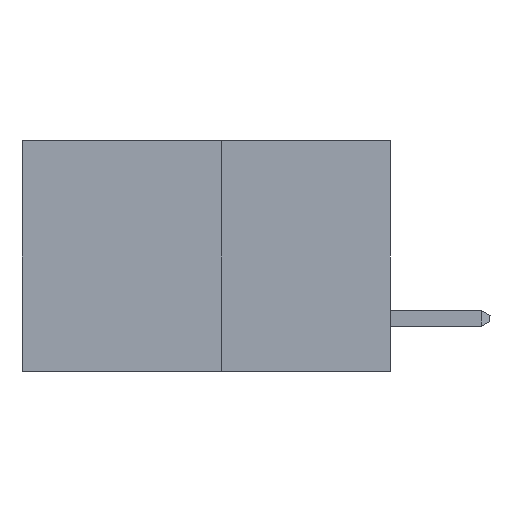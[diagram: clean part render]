
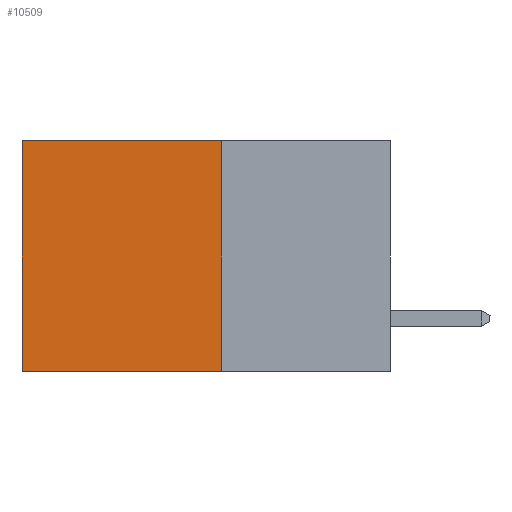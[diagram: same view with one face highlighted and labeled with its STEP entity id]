
A CAD part, left-side view. The second image highlights one B-rep face of the part: STEP entity #10509.
In plain terms, the highlighted planar face has unit normal (-1, 0, 0).
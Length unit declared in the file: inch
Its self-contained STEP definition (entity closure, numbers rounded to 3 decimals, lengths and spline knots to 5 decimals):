
#114 = CARTESIAN_POINT ( 'NONE',  ( 0.277, 0.27, -0.37 ) ) ;
#220 = EDGE_LOOP ( 'NONE', ( #13788, #3759, #4108, #1432 ) ) ;
#617 = PLANE ( 'NONE',  #11642 ) ;
#951 = CARTESIAN_POINT ( 'NONE',  ( 0.277, 0.27, -0.37 ) ) ;
#1059 = DIRECTION ( 'NONE',  ( 0., 0., -1. ) ) ;
#1062 = DIRECTION ( 'NONE',  ( 0., 1., 0. ) ) ;
#1432 = ORIENTED_EDGE ( 'NONE', *, *, #11243, .T. ) ;
#1532 = VECTOR ( 'NONE', #1059, 39.37008 ) ;
#2311 = VECTOR ( 'NONE', #1062, 39.37008 ) ;
#2806 = DIRECTION ( 'NONE',  ( 0., 1., 0. ) ) ;
#2920 = DIRECTION ( 'NONE',  ( 0., 0., -1. ) ) ;
#3384 = VERTEX_POINT ( 'NONE', #4161 ) ;
#3733 = EDGE_CURVE ( 'NONE', #11399, #3384, #7106, .T. ) ;
#3759 = ORIENTED_EDGE ( 'NONE', *, *, #3733, .F. ) ;
#4075 = VECTOR ( 'NONE', #2806, 39.37008 ) ;
#4108 = ORIENTED_EDGE ( 'NONE', *, *, #5228, .F. ) ;
#4161 = CARTESIAN_POINT ( 'NONE',  ( 0.277, 0.59, -0.37 ) ) ;
#4196 = LINE ( 'NONE', #951, #1532 ) ;
#4508 = FACE_OUTER_BOUND ( 'NONE', #220, .T. ) ;
#4796 = CARTESIAN_POINT ( 'NONE',  ( 0.277, 0.59, -0.37 ) ) ;
#5146 = CARTESIAN_POINT ( 'NONE',  ( 0.277, 0.27, -0.37 ) ) ;
#5228 = EDGE_CURVE ( 'NONE', #11792, #11399, #4196, .T. ) ;
#5358 = CARTESIAN_POINT ( 'NONE',  ( 0.277, 0.27, 0. ) ) ;
#7088 = DIRECTION ( 'NONE',  ( 0., 0., -1. ) ) ;
#7106 = LINE ( 'NONE', #9039, #4075 ) ;
#7869 = CARTESIAN_POINT ( 'NONE',  ( 0.277, 0.27, 0. ) ) ;
#8326 = LINE ( 'NONE', #7869, #2311 ) ;
#8332 = VERTEX_POINT ( 'NONE', #12880 ) ;
#8647 = VECTOR ( 'NONE', #7088, 39.37008 ) ;
#9039 = CARTESIAN_POINT ( 'NONE',  ( 0.277, 0.27, -0.37 ) ) ;
#9665 = DIRECTION ( 'NONE',  ( 1., 0., 0. ) ) ;
#10509 = ADVANCED_FACE ( 'NONE', ( #4508 ), #617, .F. ) ;
#11243 = EDGE_CURVE ( 'NONE', #11792, #8332, #8326, .T. ) ;
#11399 = VERTEX_POINT ( 'NONE', #114 ) ;
#11642 = AXIS2_PLACEMENT_3D ( 'NONE', #5146, #9665, #2920 ) ;
#11792 = VERTEX_POINT ( 'NONE', #5358 ) ;
#12676 = EDGE_CURVE ( 'NONE', #8332, #3384, #14462, .T. ) ;
#12880 = CARTESIAN_POINT ( 'NONE',  ( 0.277, 0.59, 0. ) ) ;
#13788 = ORIENTED_EDGE ( 'NONE', *, *, #12676, .T. ) ;
#14462 = LINE ( 'NONE', #4796, #8647 ) ;
